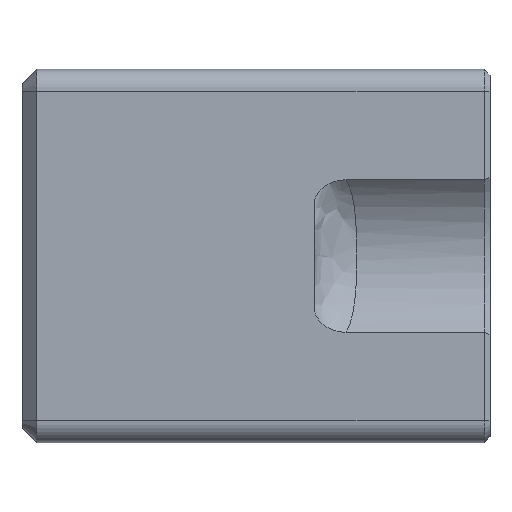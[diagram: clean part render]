
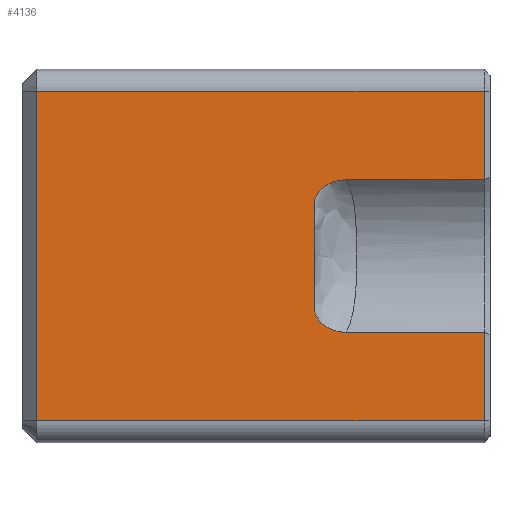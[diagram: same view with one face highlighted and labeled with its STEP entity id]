
A CAD part, front view. The second image highlights one B-rep face of the part: STEP entity #4136.
In plain terms, the highlighted planar face has unit normal (0, -1, 0).
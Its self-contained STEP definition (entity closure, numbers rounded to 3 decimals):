
#541=B_SPLINE_CURVE_WITH_KNOTS('',3,(#11925,#11926,#11927,#11928,#11929,
#11930,#11931,#11932,#11933,#11934,#11935,#11936,#11937,#11938,#11939,#11940,
#11941,#11942,#11943,#11944),.UNSPECIFIED.,.F.,.F.,(4,2,2,2,2,2,2,2,2,4),
(0.,0.,0.,0.003,0.007,
0.017,0.038,0.082,0.153,
0.23),.UNSPECIFIED.);
#542=B_SPLINE_CURVE_WITH_KNOTS('',3,(#11948,#11949,#11950,#11951,#11952,
#11953,#11954,#11955,#11956,#11957,#11958,#11959,#11960,#11961,#11962,#11963,
#11964,#11965,#11966,#11967),.UNSPECIFIED.,.F.,.F.,(4,2,2,2,2,2,2,2,2,4),
(0.,0.101,0.195,0.253,0.281,
0.294,0.3,0.303,0.303,
0.303),.UNSPECIFIED.);
#594=PLANE('',#4426);
#898=FACE_OUTER_BOUND('',#1151,.T.);
#1151=EDGE_LOOP('',(#3808,#3809,#3810,#3811,#3812,#3813,#3814,#3815,#3816,
#3817));
#1256=LINE('',#11892,#1373);
#1265=LINE('',#11914,#1382);
#1266=LINE('',#11919,#1383);
#1267=LINE('',#11923,#1384);
#1268=LINE('',#11946,#1385);
#1269=LINE('',#11968,#1386);
#1270=LINE('',#11970,#1387);
#1271=LINE('',#11971,#1388);
#1373=VECTOR('',#5004,10.);
#1382=VECTOR('',#5037,10.);
#1383=VECTOR('',#5044,10.);
#1384=VECTOR('',#5049,10.);
#1385=VECTOR('',#5050,10.);
#1386=VECTOR('',#5051,10.);
#1387=VECTOR('',#5052,10.);
#1388=VECTOR('',#5053,10.);
#1928=VERTEX_POINT('',#11879);
#1929=VERTEX_POINT('',#11884);
#1930=VERTEX_POINT('',#11891);
#1931=VERTEX_POINT('',#11910);
#1932=VERTEX_POINT('',#11918);
#1933=VERTEX_POINT('',#11922);
#1934=VERTEX_POINT('',#11924);
#1935=VERTEX_POINT('',#11945);
#1936=VERTEX_POINT('',#11947);
#1937=VERTEX_POINT('',#11969);
#2548=EDGE_CURVE('',#1929,#1930,#1256,.T.);
#2561=EDGE_CURVE('',#1931,#1928,#1265,.T.);
#2563=EDGE_CURVE('',#1930,#1932,#1266,.T.);
#2565=EDGE_CURVE('',#1929,#1933,#1267,.T.);
#2566=EDGE_CURVE('',#1934,#1933,#541,.T.);
#2567=EDGE_CURVE('',#1934,#1935,#1268,.T.);
#2568=EDGE_CURVE('',#1935,#1936,#542,.F.);
#2569=EDGE_CURVE('',#1936,#1928,#1269,.T.);
#2570=EDGE_CURVE('',#1937,#1931,#1270,.T.);
#2571=EDGE_CURVE('',#1932,#1937,#1271,.T.);
#3808=ORIENTED_EDGE('',*,*,#2548,.F.);
#3809=ORIENTED_EDGE('',*,*,#2565,.T.);
#3810=ORIENTED_EDGE('',*,*,#2566,.F.);
#3811=ORIENTED_EDGE('',*,*,#2567,.T.);
#3812=ORIENTED_EDGE('',*,*,#2568,.T.);
#3813=ORIENTED_EDGE('',*,*,#2569,.T.);
#3814=ORIENTED_EDGE('',*,*,#2561,.F.);
#3815=ORIENTED_EDGE('',*,*,#2570,.F.);
#3816=ORIENTED_EDGE('',*,*,#2571,.F.);
#3817=ORIENTED_EDGE('',*,*,#2563,.F.);
#4136=ADVANCED_FACE('',(#898),#594,.T.);
#4426=AXIS2_PLACEMENT_3D('',#11921,#5047,#5048);
#5004=DIRECTION('',(0.,0.,-1.));
#5037=DIRECTION('',(0.,0.,-1.));
#5044=DIRECTION('',(-1.,0.,0.));
#5047=DIRECTION('center_axis',(0.,-1.,0.));
#5048=DIRECTION('ref_axis',(0.,0.,1.));
#5049=DIRECTION('',(-1.,0.,0.));
#5050=DIRECTION('',(0.,0.,1.));
#5051=DIRECTION('',(1.,0.,0.));
#5052=DIRECTION('',(1.,0.,0.));
#5053=DIRECTION('',(0.,0.,1.));
#11879=CARTESIAN_POINT('',(-183.534,-11.455,5.212));
#11884=CARTESIAN_POINT('',(-183.534,-11.455,-5.212));
#11891=CARTESIAN_POINT('',(-183.534,-11.455,-11.264));
#11892=CARTESIAN_POINT('',(-183.534,-11.455,-6.128));
#11910=CARTESIAN_POINT('',(-183.534,-11.455,11.264));
#11914=CARTESIAN_POINT('',(-183.534,-11.455,-6.128));
#11918=CARTESIAN_POINT('',(-214.134,-11.455,-11.264));
#11919=CARTESIAN_POINT('',(-183.134,-11.455,-11.264));
#11921=CARTESIAN_POINT('Origin',(-183.134,-11.455,-12.256));
#11922=CARTESIAN_POINT('',(-192.977,-11.455,-5.212));
#11923=CARTESIAN_POINT('',(-183.134,-11.455,-5.212));
#11924=CARTESIAN_POINT('',(-195.134,-11.455,-3.728));
#11925=CARTESIAN_POINT('Ctrl Pts',(-195.134,-11.455,-3.728));
#11926=CARTESIAN_POINT('Ctrl Pts',(-195.134,-11.455,-3.729));
#11927=CARTESIAN_POINT('Ctrl Pts',(-195.134,-11.455,-3.729));
#11928=CARTESIAN_POINT('Ctrl Pts',(-195.134,-11.455,-3.731));
#11929=CARTESIAN_POINT('Ctrl Pts',(-195.134,-11.455,-3.732));
#11930=CARTESIAN_POINT('Ctrl Pts',(-195.133,-11.455,-3.741));
#11931=CARTESIAN_POINT('Ctrl Pts',(-195.133,-11.455,-3.75));
#11932=CARTESIAN_POINT('Ctrl Pts',(-195.13,-11.455,-3.775));
#11933=CARTESIAN_POINT('Ctrl Pts',(-195.127,-11.455,-3.792));
#11934=CARTESIAN_POINT('Ctrl Pts',(-195.115,-11.455,-3.847));
#11935=CARTESIAN_POINT('Ctrl Pts',(-195.105,-11.455,-3.884));
#11936=CARTESIAN_POINT('Ctrl Pts',(-195.067,-11.455,-3.997));
#11937=CARTESIAN_POINT('Ctrl Pts',(-195.033,-11.455,-4.071));
#11938=CARTESIAN_POINT('Ctrl Pts',(-194.914,-11.455,-4.289));
#11939=CARTESIAN_POINT('Ctrl Pts',(-194.809,-11.455,
-4.425));
#11940=CARTESIAN_POINT('Ctrl Pts',(-194.496,-11.455,
-4.738));
#11941=CARTESIAN_POINT('Ctrl Pts',(-194.251,-11.455,-4.903));
#11942=CARTESIAN_POINT('Ctrl Pts',(-193.651,-11.455,-5.15));
#11943=CARTESIAN_POINT('Ctrl Pts',(-193.316,-11.455,-5.212));
#11944=CARTESIAN_POINT('Ctrl Pts',(-192.977,-11.455,-5.212));
#11945=CARTESIAN_POINT('',(-195.134,-11.455,3.728));
#11946=CARTESIAN_POINT('',(-195.134,-11.455,-6.128));
#11947=CARTESIAN_POINT('',(-192.977,-11.455,5.212));
#11948=CARTESIAN_POINT('Ctrl Pts',(-192.977,-11.455,5.212));
#11949=CARTESIAN_POINT('Ctrl Pts',(-193.316,-11.455,5.212));
#11950=CARTESIAN_POINT('Ctrl Pts',(-193.651,-11.455,5.15));
#11951=CARTESIAN_POINT('Ctrl Pts',(-194.251,-11.455,4.903));
#11952=CARTESIAN_POINT('Ctrl Pts',(-194.496,-11.455,
4.738));
#11953=CARTESIAN_POINT('Ctrl Pts',(-194.809,-11.455,
4.425));
#11954=CARTESIAN_POINT('Ctrl Pts',(-194.914,-11.455,4.289));
#11955=CARTESIAN_POINT('Ctrl Pts',(-195.034,-11.455,4.071));
#11956=CARTESIAN_POINT('Ctrl Pts',(-195.067,-11.455,3.997));
#11957=CARTESIAN_POINT('Ctrl Pts',(-195.105,-11.455,3.884));
#11958=CARTESIAN_POINT('Ctrl Pts',(-195.115,-11.455,3.847));
#11959=CARTESIAN_POINT('Ctrl Pts',(-195.127,-11.455,3.792));
#11960=CARTESIAN_POINT('Ctrl Pts',(-195.13,-11.455,3.775));
#11961=CARTESIAN_POINT('Ctrl Pts',(-195.133,-11.455,3.75));
#11962=CARTESIAN_POINT('Ctrl Pts',(-195.133,-11.455,3.741));
#11963=CARTESIAN_POINT('Ctrl Pts',(-195.134,-11.455,3.732));
#11964=CARTESIAN_POINT('Ctrl Pts',(-195.134,-11.455,3.731));
#11965=CARTESIAN_POINT('Ctrl Pts',(-195.134,-11.455,3.729));
#11966=CARTESIAN_POINT('Ctrl Pts',(-195.134,-11.455,3.728));
#11967=CARTESIAN_POINT('Ctrl Pts',(-195.134,-11.455,3.728));
#11968=CARTESIAN_POINT('',(-183.134,-11.455,5.212));
#11969=CARTESIAN_POINT('',(-214.134,-11.455,11.264));
#11970=CARTESIAN_POINT('',(-183.134,-11.455,11.264));
#11971=CARTESIAN_POINT('',(-214.134,-11.455,-6.128));
